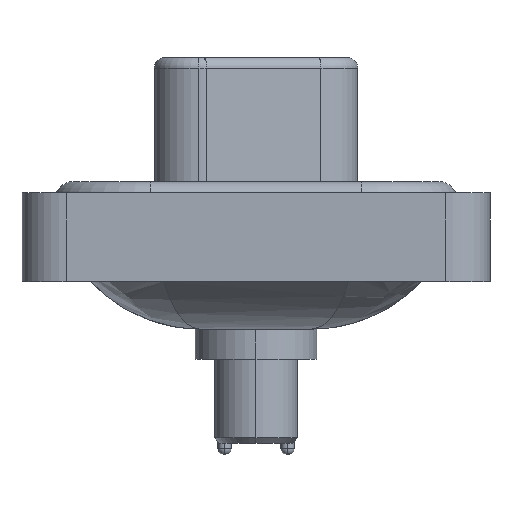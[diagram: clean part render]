
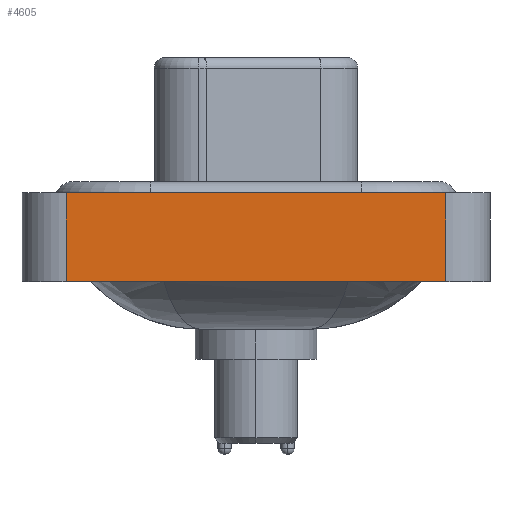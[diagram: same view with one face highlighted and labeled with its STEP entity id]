
A CAD part, left-side view. The second image highlights one B-rep face of the part: STEP entity #4605.
In plain terms, the highlighted planar face has unit normal (-1, 0, 0).
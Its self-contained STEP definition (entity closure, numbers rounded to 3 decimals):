
#320 = VECTOR ( 'NONE', #7393, 1000. ) ;
#819 = AXIS2_PLACEMENT_3D ( 'NONE', #2455, #2562, #886 ) ;
#886 = DIRECTION ( 'NONE',  ( 0., 0., 1. ) ) ;
#1133 = VERTEX_POINT ( 'NONE', #9208 ) ;
#1442 = VECTOR ( 'NONE', #14839, 1000. ) ;
#1920 = EDGE_CURVE ( 'NONE', #9890, #14165, #7599, .T. ) ;
#1989 = ORIENTED_EDGE ( 'NONE', *, *, #9112, .T. ) ;
#2455 = CARTESIAN_POINT ( 'NONE',  ( -7.35, -8.55, -3.6 ) ) ;
#2562 = DIRECTION ( 'NONE',  ( -1., 0., 0. ) ) ;
#2830 = EDGE_CURVE ( 'NONE', #1133, #7916, #5641, .T. ) ;
#3130 = CARTESIAN_POINT ( 'NONE',  ( -7.35, -8.55, -3.6 ) ) ;
#3782 = CARTESIAN_POINT ( 'NONE',  ( -7.35, -8.55, -3.6 ) ) ;
#4500 = EDGE_LOOP ( 'NONE', ( #1989, #17962, #4755, #19086 ) ) ;
#4605 = ADVANCED_FACE ( 'NONE', ( #5300 ), #18031, .T. ) ;
#4755 = ORIENTED_EDGE ( 'NONE', *, *, #10643, .F. ) ;
#5010 = CARTESIAN_POINT ( 'NONE',  ( -7.35, -8.55, 0.4 ) ) ;
#5300 = FACE_OUTER_BOUND ( 'NONE', #4500, .T. ) ;
#5641 = LINE ( 'NONE', #16277, #18405 ) ;
#5939 = VECTOR ( 'NONE', #11170, 1000. ) ;
#7393 = DIRECTION ( 'NONE',  ( 0., -1., 0. ) ) ;
#7599 = LINE ( 'NONE', #13737, #320 ) ;
#7916 = VERTEX_POINT ( 'NONE', #5010 ) ;
#8303 = LINE ( 'NONE', #3782, #1442 ) ;
#9112 = EDGE_CURVE ( 'NONE', #14165, #7916, #8303, .T. ) ;
#9208 = CARTESIAN_POINT ( 'NONE',  ( -7.35, 8.55, 0.4 ) ) ;
#9597 = CARTESIAN_POINT ( 'NONE',  ( -7.35, 8.55, -3.6 ) ) ;
#9890 = VERTEX_POINT ( 'NONE', #9597 ) ;
#10522 = DIRECTION ( 'NONE',  ( 0., -1., 0. ) ) ;
#10643 = EDGE_CURVE ( 'NONE', #9890, #1133, #12753, .T. ) ;
#11170 = DIRECTION ( 'NONE',  ( 0., 0., 1. ) ) ;
#12753 = LINE ( 'NONE', #19114, #5939 ) ;
#13737 = CARTESIAN_POINT ( 'NONE',  ( -7.35, -8.55, -3.6 ) ) ;
#14165 = VERTEX_POINT ( 'NONE', #3130 ) ;
#14839 = DIRECTION ( 'NONE',  ( 0., 0., 1. ) ) ;
#16277 = CARTESIAN_POINT ( 'NONE',  ( -7.35, -8.55, 0.4 ) ) ;
#17962 = ORIENTED_EDGE ( 'NONE', *, *, #2830, .F. ) ;
#18031 = PLANE ( 'NONE',  #819 ) ;
#18405 = VECTOR ( 'NONE', #10522, 1000. ) ;
#19086 = ORIENTED_EDGE ( 'NONE', *, *, #1920, .T. ) ;
#19114 = CARTESIAN_POINT ( 'NONE',  ( -7.35, 8.55, -3.6 ) ) ;
